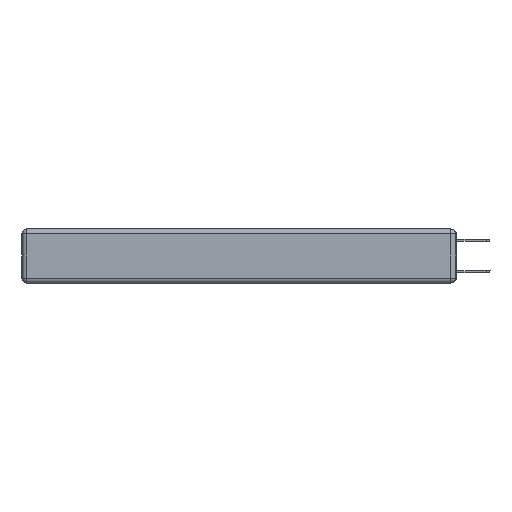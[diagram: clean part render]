
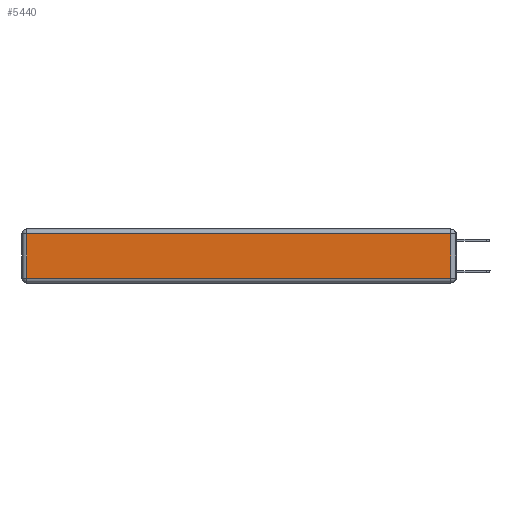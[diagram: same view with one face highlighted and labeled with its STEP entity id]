
A CAD part, left-side view. The second image highlights one B-rep face of the part: STEP entity #5440.
In plain terms, the highlighted planar face has unit normal (-1, 0, 0).
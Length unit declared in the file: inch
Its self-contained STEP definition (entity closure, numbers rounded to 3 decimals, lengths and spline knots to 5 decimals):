
#25 = LINE ( 'NONE', #13559, #11394 ) ;
#414 = EDGE_LOOP ( 'NONE', ( #13916, #13981, #10024, #17982 ) ) ;
#1087 = LINE ( 'NONE', #15637, #9977 ) ;
#1622 = EDGE_CURVE ( 'NONE', #14359, #11651, #17229, .T. ) ;
#3124 = FACE_OUTER_BOUND ( 'NONE', #414, .T. ) ;
#4805 = EDGE_CURVE ( 'NONE', #11651, #4966, #25, .T. ) ;
#4925 = CARTESIAN_POINT ( 'NONE',  ( 0., 0.03, -0.313 ) ) ;
#4966 = VERTEX_POINT ( 'NONE', #17084 ) ;
#5440 = ADVANCED_FACE ( 'NONE', ( #3124 ), #15762, .T. ) ;
#6269 = VECTOR ( 'NONE', #12608, 39.37008 ) ;
#6658 = CARTESIAN_POINT ( 'NONE',  ( 0., 2.75, -0.03 ) ) ;
#7767 = EDGE_CURVE ( 'NONE', #15673, #14359, #17091, .T. ) ;
#7949 = CARTESIAN_POINT ( 'NONE',  ( 0., 0., -0.343 ) ) ;
#7968 = VECTOR ( 'NONE', #16806, 39.37008 ) ;
#8664 = CARTESIAN_POINT ( 'NONE',  ( 0., 0.03, -0.03 ) ) ;
#9779 = AXIS2_PLACEMENT_3D ( 'NONE', #7949, #18813, #12714 ) ;
#9845 = DIRECTION ( 'NONE',  ( 0., -1., 0. ) ) ;
#9977 = VECTOR ( 'NONE', #9845, 39.37008 ) ;
#10024 = ORIENTED_EDGE ( 'NONE', *, *, #1622, .T. ) ;
#11394 = VECTOR ( 'NONE', #17983, 39.37008 ) ;
#11651 = VERTEX_POINT ( 'NONE', #14972 ) ;
#12608 = DIRECTION ( 'NONE',  ( 0., 1., 0. ) ) ;
#12714 = DIRECTION ( 'NONE',  ( 0., 0., 1. ) ) ;
#13559 = CARTESIAN_POINT ( 'NONE',  ( 0., 2.72, -0.343 ) ) ;
#13916 = ORIENTED_EDGE ( 'NONE', *, *, #16736, .T. ) ;
#13981 = ORIENTED_EDGE ( 'NONE', *, *, #7767, .T. ) ;
#14146 = CARTESIAN_POINT ( 'NONE',  ( 0., 0.03, -0.343 ) ) ;
#14359 = VERTEX_POINT ( 'NONE', #8664 ) ;
#14972 = CARTESIAN_POINT ( 'NONE',  ( 0., 2.72, -0.03 ) ) ;
#15637 = CARTESIAN_POINT ( 'NONE',  ( 0., 0., -0.313 ) ) ;
#15673 = VERTEX_POINT ( 'NONE', #4925 ) ;
#15762 = PLANE ( 'NONE',  #9779 ) ;
#16736 = EDGE_CURVE ( 'NONE', #4966, #15673, #1087, .T. ) ;
#16806 = DIRECTION ( 'NONE',  ( 0., 0., 1. ) ) ;
#17084 = CARTESIAN_POINT ( 'NONE',  ( 0., 2.72, -0.313 ) ) ;
#17091 = LINE ( 'NONE', #14146, #7968 ) ;
#17229 = LINE ( 'NONE', #6658, #6269 ) ;
#17982 = ORIENTED_EDGE ( 'NONE', *, *, #4805, .T. ) ;
#17983 = DIRECTION ( 'NONE',  ( 0., 0., -1. ) ) ;
#18813 = DIRECTION ( 'NONE',  ( -1., 0., 0. ) ) ;
